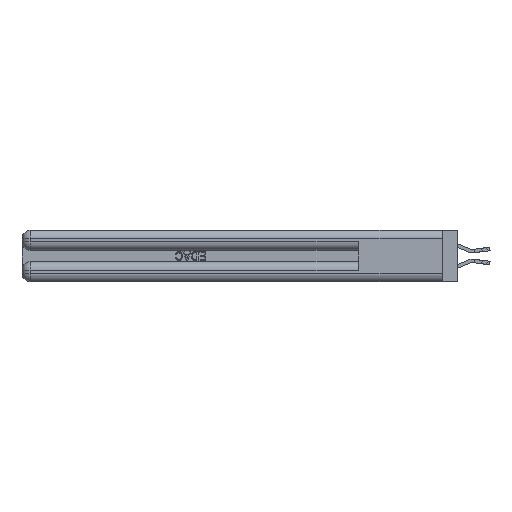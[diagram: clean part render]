
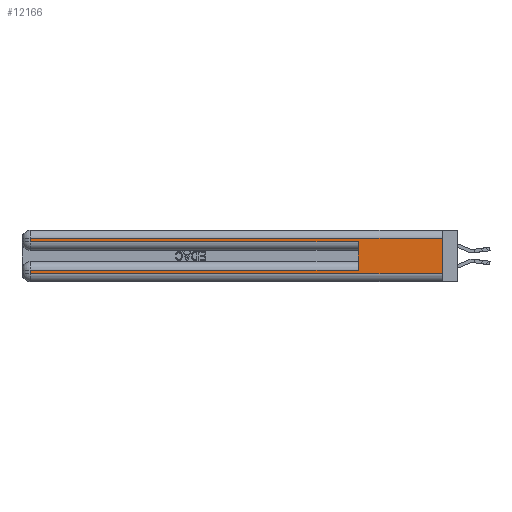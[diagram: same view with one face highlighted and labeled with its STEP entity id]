
A CAD part, left-side view. The second image highlights one B-rep face of the part: STEP entity #12166.
In plain terms, the highlighted planar face has unit normal (-1, 0, 0).
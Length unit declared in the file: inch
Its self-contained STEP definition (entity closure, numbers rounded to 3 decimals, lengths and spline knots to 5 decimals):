
#1242 = CARTESIAN_POINT ( 'NONE',  ( 0., 0., 0.285 ) ) ;
#1344 = CARTESIAN_POINT ( 'NONE',  ( 0., 0., 0.37 ) ) ;
#2000 = DIRECTION ( 'NONE',  ( 0., 0., 1. ) ) ;
#2295 = VECTOR ( 'NONE', #25566, 39.37008 ) ;
#3581 = EDGE_CURVE ( 'NONE', #24030, #39250, #39230, .T. ) ;
#3636 = EDGE_LOOP ( 'NONE', ( #16466, #31064, #12434, #31760, #16184, #15268, #7645, #22579 ) ) ;
#3703 = VECTOR ( 'NONE', #15394, 39.37008 ) ;
#5137 = CARTESIAN_POINT ( 'NONE',  ( 0., 0.6, 0.085 ) ) ;
#6682 = LINE ( 'NONE', #7612, #33275 ) ;
#6795 = DIRECTION ( 'NONE',  ( 0., 0., -1. ) ) ;
#6868 = CARTESIAN_POINT ( 'NONE',  ( 0., 0., 0.31 ) ) ;
#6948 = VECTOR ( 'NONE', #35041, 39.37008 ) ;
#7612 = CARTESIAN_POINT ( 'NONE',  ( 0., 0., 0.06 ) ) ;
#7645 = ORIENTED_EDGE ( 'NONE', *, *, #28435, .T. ) ;
#8467 = LINE ( 'NONE', #32037, #34560 ) ;
#8719 = CARTESIAN_POINT ( 'NONE',  ( 0., 0., 0.085 ) ) ;
#8773 = VERTEX_POINT ( 'NONE', #33333 ) ;
#9784 = VERTEX_POINT ( 'NONE', #17747 ) ;
#11232 = CARTESIAN_POINT ( 'NONE',  ( 0., 2.94, 0.31 ) ) ;
#11300 = LINE ( 'NONE', #1344, #2295 ) ;
#11393 = VERTEX_POINT ( 'NONE', #17333 ) ;
#11888 = EDGE_CURVE ( 'NONE', #23037, #18580, #35609, .T. ) ;
#12166 = ADVANCED_FACE ( 'NONE', ( #26076 ), #31195, .F. ) ;
#12434 = ORIENTED_EDGE ( 'NONE', *, *, #19798, .T. ) ;
#12891 = EDGE_CURVE ( 'NONE', #23037, #39250, #16154, .T. ) ;
#13378 = CARTESIAN_POINT ( 'NONE',  ( 0., 0.6, 0.285 ) ) ;
#14817 = DIRECTION ( 'NONE',  ( 0., 1., 0. ) ) ;
#15268 = ORIENTED_EDGE ( 'NONE', *, *, #11888, .T. ) ;
#15394 = DIRECTION ( 'NONE',  ( 0., 1., 0. ) ) ;
#16154 = LINE ( 'NONE', #35549, #30378 ) ;
#16184 = ORIENTED_EDGE ( 'NONE', *, *, #12891, .F. ) ;
#16362 = DIRECTION ( 'NONE',  ( 0., 0., -1. ) ) ;
#16466 = ORIENTED_EDGE ( 'NONE', *, *, #36860, .F. ) ;
#17333 = CARTESIAN_POINT ( 'NONE',  ( 0., 0., 0.06 ) ) ;
#17747 = CARTESIAN_POINT ( 'NONE',  ( 0., 2.94, 0.06 ) ) ;
#18159 = VECTOR ( 'NONE', #6795, 39.37008 ) ;
#18580 = VERTEX_POINT ( 'NONE', #24902 ) ;
#19523 = DIRECTION ( 'NONE',  ( 1., 0., 0. ) ) ;
#19798 = EDGE_CURVE ( 'NONE', #27141, #24030, #26170, .T. ) ;
#20082 = DIRECTION ( 'NONE',  ( 0., 0., -1. ) ) ;
#22579 = ORIENTED_EDGE ( 'NONE', *, *, #35358, .T. ) ;
#23037 = VERTEX_POINT ( 'NONE', #5137 ) ;
#24030 = VERTEX_POINT ( 'NONE', #37274 ) ;
#24760 = EDGE_CURVE ( 'NONE', #8773, #27141, #30747, .T. ) ;
#24902 = CARTESIAN_POINT ( 'NONE',  ( 0., 2.94, 0.085 ) ) ;
#25566 = DIRECTION ( 'NONE',  ( 0., 0., -1. ) ) ;
#25610 = VECTOR ( 'NONE', #14817, 39.37008 ) ;
#26076 = FACE_OUTER_BOUND ( 'NONE', #3636, .T. ) ;
#26170 = LINE ( 'NONE', #33857, #18159 ) ;
#27141 = VERTEX_POINT ( 'NONE', #11232 ) ;
#28275 = CARTESIAN_POINT ( 'NONE',  ( 0., 0., 0.37 ) ) ;
#28435 = EDGE_CURVE ( 'NONE', #18580, #9784, #8467, .T. ) ;
#28933 = DIRECTION ( 'NONE',  ( 0., -1., 0. ) ) ;
#30378 = VECTOR ( 'NONE', #2000, 39.37008 ) ;
#30747 = LINE ( 'NONE', #6868, #3703 ) ;
#31064 = ORIENTED_EDGE ( 'NONE', *, *, #24760, .T. ) ;
#31195 = PLANE ( 'NONE',  #37631 ) ;
#31760 = ORIENTED_EDGE ( 'NONE', *, *, #3581, .T. ) ;
#32037 = CARTESIAN_POINT ( 'NONE',  ( 0., 2.94, 0.37 ) ) ;
#33275 = VECTOR ( 'NONE', #28933, 39.37008 ) ;
#33333 = CARTESIAN_POINT ( 'NONE',  ( 0., 0., 0.31 ) ) ;
#33857 = CARTESIAN_POINT ( 'NONE',  ( 0., 2.94, 0.37 ) ) ;
#34560 = VECTOR ( 'NONE', #20082, 39.37008 ) ;
#35041 = DIRECTION ( 'NONE',  ( 0., -1., 0. ) ) ;
#35358 = EDGE_CURVE ( 'NONE', #9784, #11393, #6682, .T. ) ;
#35549 = CARTESIAN_POINT ( 'NONE',  ( 0., 0.6, 0.145 ) ) ;
#35609 = LINE ( 'NONE', #8719, #25610 ) ;
#36860 = EDGE_CURVE ( 'NONE', #8773, #11393, #11300, .T. ) ;
#37274 = CARTESIAN_POINT ( 'NONE',  ( 0., 2.94, 0.285 ) ) ;
#37631 = AXIS2_PLACEMENT_3D ( 'NONE', #28275, #19523, #16362 ) ;
#39230 = LINE ( 'NONE', #1242, #6948 ) ;
#39250 = VERTEX_POINT ( 'NONE', #13378 ) ;
